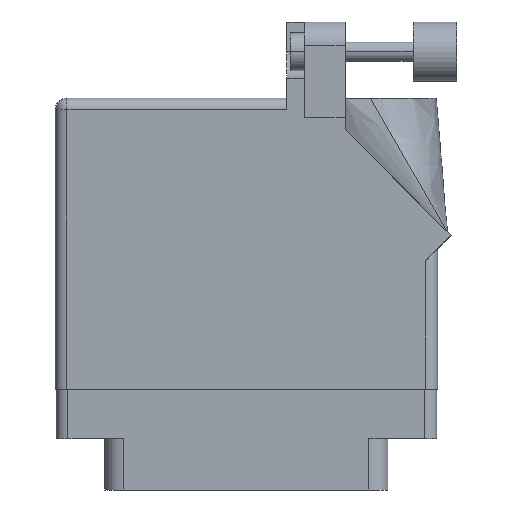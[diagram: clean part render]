
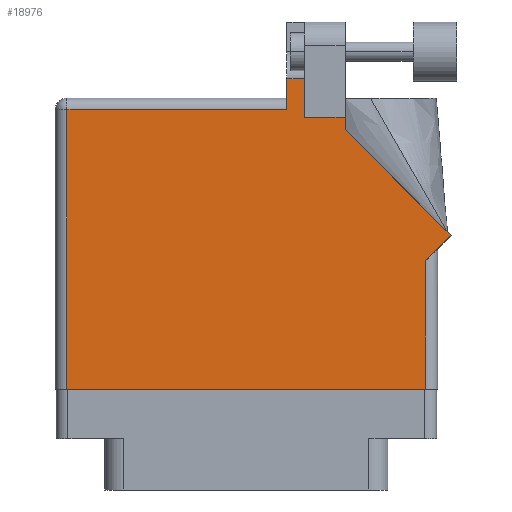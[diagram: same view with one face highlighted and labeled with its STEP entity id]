
A CAD part, front view. The second image highlights one B-rep face of the part: STEP entity #18976.
In plain terms, the highlighted face is planar.
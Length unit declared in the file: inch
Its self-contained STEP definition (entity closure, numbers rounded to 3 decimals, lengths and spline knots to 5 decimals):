
#518 = VERTEX_POINT ( 'NONE', #6975 ) ;
#767 = EDGE_CURVE ( 'NONE', #518, #13818, #15958, .T. ) ;
#897 = LINE ( 'NONE', #21790, #22276 ) ;
#1060 = VECTOR ( 'NONE', #25713, 39.37008 ) ;
#1558 = VECTOR ( 'NONE', #29729, 39.37008 ) ;
#2060 = VECTOR ( 'NONE', #16010, 39.37008 ) ;
#2264 = VERTEX_POINT ( 'NONE', #30952 ) ;
#2807 = ORIENTED_EDGE ( 'NONE', *, *, #21779, .T. ) ;
#2832 = CARTESIAN_POINT ( 'NONE',  ( 1.217, 1.6315, 0. ) ) ;
#3331 = EDGE_CURVE ( 'NONE', #2264, #34079, #32486, .T. ) ;
#3495 = ORIENTED_EDGE ( 'NONE', *, *, #32133, .T. ) ;
#3597 = VECTOR ( 'NONE', #27032, 39.37008 ) ;
#4168 = DIRECTION ( 'NONE',  ( 0., -1., 0. ) ) ;
#4536 = ORIENTED_EDGE ( 'NONE', *, *, #17028, .T. ) ;
#4569 = DIRECTION ( 'NONE',  ( -1., 0., 0. ) ) ;
#5302 = EDGE_LOOP ( 'NONE', ( #22762, #21627, #12818, #29227, #28706, #2807, #3495, #16729, #27103, #26202, #4536 ) ) ;
#5667 = DIRECTION ( 'NONE',  ( 0., 1., 0. ) ) ;
#6496 = VECTOR ( 'NONE', #22212, 39.37008 ) ;
#6831 = CARTESIAN_POINT ( 'NONE',  ( 1.524, 1.36442, 0. ) ) ;
#6925 = DIRECTION ( 'NONE',  ( 0.707, 0.707, 0. ) ) ;
#6975 = CARTESIAN_POINT ( 'NONE',  ( 1.311, 1.43, 0. ) ) ;
#7851 = CARTESIAN_POINT ( 'NONE',  ( 0., 0., 0. ) ) ;
#8180 = EDGE_CURVE ( 'NONE', #13818, #14536, #31327, .T. ) ;
#8295 = CARTESIAN_POINT ( 'NONE',  ( 0.062, 1.468, 0. ) ) ;
#9444 = LINE ( 'NONE', #12248, #12860 ) ;
#9514 = LINE ( 'NONE', #6831, #14630 ) ;
#10466 = CARTESIAN_POINT ( 'NONE',  ( 1.217, 1.53, 0. ) ) ;
#10553 = DIRECTION ( 'NONE',  ( 0., 0., -1. ) ) ;
#11155 = CARTESIAN_POINT ( 'NONE',  ( 2.08071, 0.80771, 0. ) ) ;
#11247 = LINE ( 'NONE', #20585, #1060 ) ;
#12248 = CARTESIAN_POINT ( 'NONE',  ( 2.01, 0.737, 0. ) ) ;
#12280 = DIRECTION ( 'NONE',  ( 0., 1., 0. ) ) ;
#12818 = ORIENTED_EDGE ( 'NONE', *, *, #23513, .T. ) ;
#12860 = VECTOR ( 'NONE', #6925, 39.37008 ) ;
#13143 = VECTOR ( 'NONE', #4168, 39.37008 ) ;
#13818 = VERTEX_POINT ( 'NONE', #33151 ) ;
#14122 = FACE_OUTER_BOUND ( 'NONE', #5302, .T. ) ;
#14536 = VERTEX_POINT ( 'NONE', #2832 ) ;
#14630 = VECTOR ( 'NONE', #12280, 39.37008 ) ;
#14937 = VERTEX_POINT ( 'NONE', #31816 ) ;
#15405 = VERTEX_POINT ( 'NONE', #32299 ) ;
#15578 = VERTEX_POINT ( 'NONE', #19970 ) ;
#15958 = LINE ( 'NONE', #32603, #3597 ) ;
#16010 = DIRECTION ( 'NONE',  ( 0., -1., 0. ) ) ;
#16092 = LINE ( 'NONE', #7851, #1558 ) ;
#16577 = LINE ( 'NONE', #10466, #2060 ) ;
#16729 = ORIENTED_EDGE ( 'NONE', *, *, #31301, .T. ) ;
#17028 = EDGE_CURVE ( 'NONE', #18852, #518, #11247, .T. ) ;
#18705 = CARTESIAN_POINT ( 'NONE',  ( 1.524, 1.36442, 0. ) ) ;
#18852 = VERTEX_POINT ( 'NONE', #23419 ) ;
#18976 = ADVANCED_FACE ( 'NONE', ( #14122 ), #21483, .F. ) ;
#19376 = AXIS2_PLACEMENT_3D ( 'NONE', #26984, #10553, #29387 ) ;
#19669 = DIRECTION ( 'NONE',  ( -1., 0., 0. ) ) ;
#19970 = CARTESIAN_POINT ( 'NONE',  ( 1.948, 0., 0. ) ) ;
#20585 = CARTESIAN_POINT ( 'NONE',  ( 1.524, 1.43, 0. ) ) ;
#21483 = PLANE ( 'NONE',  #19376 ) ;
#21627 = ORIENTED_EDGE ( 'NONE', *, *, #8180, .T. ) ;
#21779 = EDGE_CURVE ( 'NONE', #23634, #15578, #16092, .T. ) ;
#21790 = CARTESIAN_POINT ( 'NONE',  ( 1.948, 0.737, 0. ) ) ;
#22212 = DIRECTION ( 'NONE',  ( -0.707, 0.707, 0. ) ) ;
#22260 = VERTEX_POINT ( 'NONE', #18705 ) ;
#22276 = VECTOR ( 'NONE', #5667, 39.37008 ) ;
#22638 = CARTESIAN_POINT ( 'NONE',  ( 0., 1.468, 0. ) ) ;
#22762 = ORIENTED_EDGE ( 'NONE', *, *, #767, .T. ) ;
#23419 = CARTESIAN_POINT ( 'NONE',  ( 1.524, 1.43, 0. ) ) ;
#23513 = EDGE_CURVE ( 'NONE', #14536, #2264, #16577, .T. ) ;
#23634 = VERTEX_POINT ( 'NONE', #35331 ) ;
#25253 = VECTOR ( 'NONE', #19669, 39.37008 ) ;
#25713 = DIRECTION ( 'NONE',  ( -1., 0., 0. ) ) ;
#26202 = ORIENTED_EDGE ( 'NONE', *, *, #27172, .T. ) ;
#26984 = CARTESIAN_POINT ( 'NONE',  ( 0., 1.53, 0. ) ) ;
#27032 = DIRECTION ( 'NONE',  ( 0., 1., 0. ) ) ;
#27103 = ORIENTED_EDGE ( 'NONE', *, *, #27542, .T. ) ;
#27172 = EDGE_CURVE ( 'NONE', #22260, #18852, #9514, .T. ) ;
#27542 = EDGE_CURVE ( 'NONE', #14937, #22260, #32959, .T. ) ;
#28706 = ORIENTED_EDGE ( 'NONE', *, *, #33578, .T. ) ;
#29227 = ORIENTED_EDGE ( 'NONE', *, *, #3331, .T. ) ;
#29387 = DIRECTION ( 'NONE',  ( -1., 0., 0. ) ) ;
#29729 = DIRECTION ( 'NONE',  ( 1., 0., 0. ) ) ;
#29886 = LINE ( 'NONE', #31038, #13143 ) ;
#30952 = CARTESIAN_POINT ( 'NONE',  ( 1.217, 1.468, 0. ) ) ;
#31038 = CARTESIAN_POINT ( 'NONE',  ( 0.062, 0., 0. ) ) ;
#31301 = EDGE_CURVE ( 'NONE', #15405, #14937, #9444, .T. ) ;
#31327 = LINE ( 'NONE', #34522, #33001 ) ;
#31816 = CARTESIAN_POINT ( 'NONE',  ( 2.08071, 0.80771, 0. ) ) ;
#32133 = EDGE_CURVE ( 'NONE', #15578, #15405, #897, .T. ) ;
#32299 = CARTESIAN_POINT ( 'NONE',  ( 1.948, 0.675, 0. ) ) ;
#32486 = LINE ( 'NONE', #22638, #25253 ) ;
#32603 = CARTESIAN_POINT ( 'NONE',  ( 1.311, 1.43, 0. ) ) ;
#32959 = LINE ( 'NONE', #11155, #6496 ) ;
#33001 = VECTOR ( 'NONE', #4569, 39.37008 ) ;
#33151 = CARTESIAN_POINT ( 'NONE',  ( 1.311, 1.6315, 0. ) ) ;
#33578 = EDGE_CURVE ( 'NONE', #34079, #23634, #29886, .T. ) ;
#34079 = VERTEX_POINT ( 'NONE', #8295 ) ;
#34522 = CARTESIAN_POINT ( 'NONE',  ( 1.64177, 1.6315, 0. ) ) ;
#35331 = CARTESIAN_POINT ( 'NONE',  ( 0.062, 0., 0. ) ) ;
